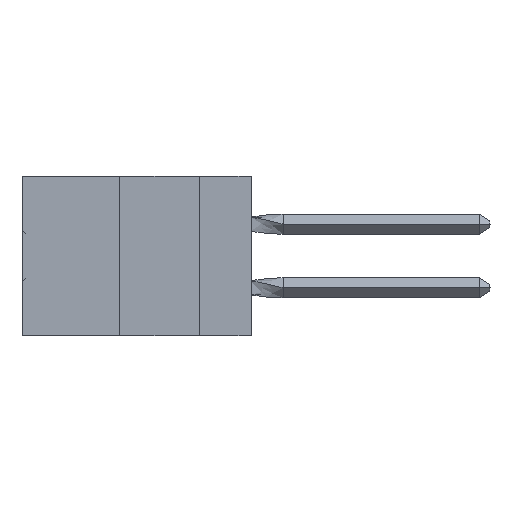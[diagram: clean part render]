
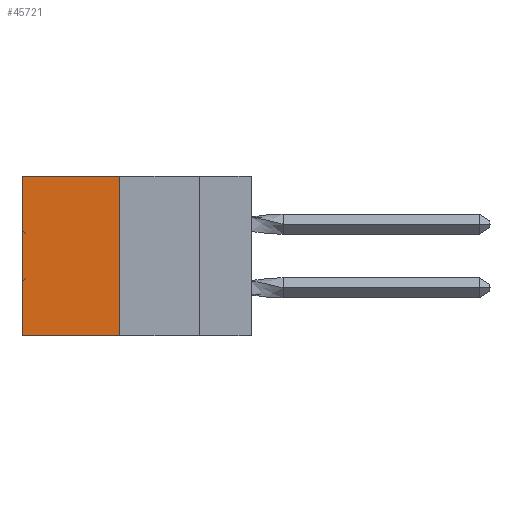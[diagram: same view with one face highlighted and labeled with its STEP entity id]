
A CAD part, left-side view. The second image highlights one B-rep face of the part: STEP entity #45721.
In plain terms, the highlighted planar face has unit normal (-1, 0, 0).
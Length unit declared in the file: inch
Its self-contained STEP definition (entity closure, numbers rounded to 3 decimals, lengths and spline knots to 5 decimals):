
#273 = DIRECTION ( 'NONE',  ( 0., 1., 0. ) ) ;
#495 = EDGE_LOOP ( 'NONE', ( #12061, #17282, #35702, #37282 ) ) ;
#811 = CARTESIAN_POINT ( 'NONE',  ( 0.305, 0.413, -0.5 ) ) ;
#7697 = VERTEX_POINT ( 'NONE', #36995 ) ;
#8703 = DIRECTION ( 'NONE',  ( 0., 0., -1. ) ) ;
#9334 = CARTESIAN_POINT ( 'NONE',  ( 0.305, 0.413, -0.5 ) ) ;
#10677 = AXIS2_PLACEMENT_3D ( 'NONE', #9334, #53514, #27098 ) ;
#10783 = VECTOR ( 'NONE', #8703, 39.37008 ) ;
#10932 = EDGE_CURVE ( 'NONE', #7697, #36066, #12956, .T. ) ;
#11012 = CARTESIAN_POINT ( 'NONE',  ( 0.305, 0.413, -0.5 ) ) ;
#11680 = EDGE_CURVE ( 'NONE', #7697, #21460, #50748, .T. ) ;
#12061 = ORIENTED_EDGE ( 'NONE', *, *, #20542, .T. ) ;
#12956 = LINE ( 'NONE', #11012, #51600 ) ;
#15406 = LINE ( 'NONE', #811, #29957 ) ;
#17282 = ORIENTED_EDGE ( 'NONE', *, *, #27963, .F. ) ;
#18444 = CARTESIAN_POINT ( 'NONE',  ( 0.305, 0.413, -0.5 ) ) ;
#18737 = CARTESIAN_POINT ( 'NONE',  ( 0.305, 0.72, 0. ) ) ;
#19906 = DIRECTION ( 'NONE',  ( 0., 0., -1. ) ) ;
#20542 = EDGE_CURVE ( 'NONE', #21460, #29441, #29451, .T. ) ;
#21460 = VERTEX_POINT ( 'NONE', #18737 ) ;
#22888 = FACE_OUTER_BOUND ( 'NONE', #495, .T. ) ;
#24834 = CARTESIAN_POINT ( 'NONE',  ( 0.305, 0.413, 0. ) ) ;
#27098 = DIRECTION ( 'NONE',  ( 0., 0., -1. ) ) ;
#27963 = EDGE_CURVE ( 'NONE', #36066, #29441, #15406, .T. ) ;
#28896 = DIRECTION ( 'NONE',  ( 0., 1., 0. ) ) ;
#29441 = VERTEX_POINT ( 'NONE', #56834 ) ;
#29451 = LINE ( 'NONE', #55102, #10783 ) ;
#29957 = VECTOR ( 'NONE', #273, 39.37008 ) ;
#35702 = ORIENTED_EDGE ( 'NONE', *, *, #10932, .F. ) ;
#36066 = VERTEX_POINT ( 'NONE', #18444 ) ;
#36995 = CARTESIAN_POINT ( 'NONE',  ( 0.305, 0.413, 0. ) ) ;
#37282 = ORIENTED_EDGE ( 'NONE', *, *, #11680, .T. ) ;
#45721 = ADVANCED_FACE ( 'NONE', ( #22888 ), #49641, .F. ) ;
#49641 = PLANE ( 'NONE',  #10677 ) ;
#50748 = LINE ( 'NONE', #24834, #53529 ) ;
#51600 = VECTOR ( 'NONE', #19906, 39.37008 ) ;
#53514 = DIRECTION ( 'NONE',  ( 1., 0., 0. ) ) ;
#53529 = VECTOR ( 'NONE', #28896, 39.37008 ) ;
#55102 = CARTESIAN_POINT ( 'NONE',  ( 0.305, 0.72, -0.5 ) ) ;
#56834 = CARTESIAN_POINT ( 'NONE',  ( 0.305, 0.72, -0.5 ) ) ;
